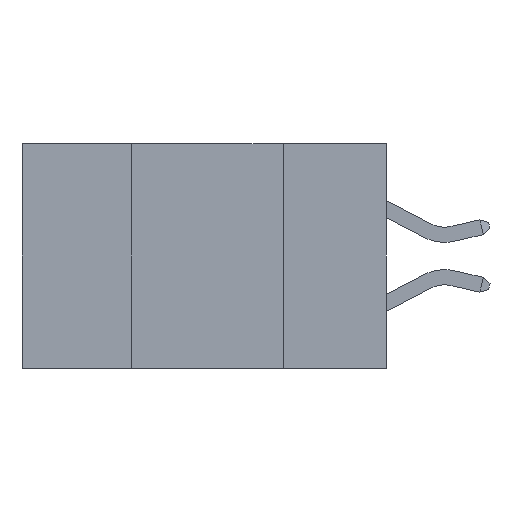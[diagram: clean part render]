
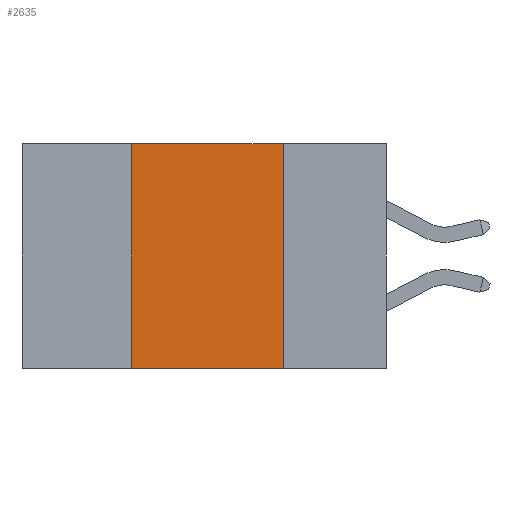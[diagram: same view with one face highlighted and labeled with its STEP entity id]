
A CAD part, left-side view. The second image highlights one B-rep face of the part: STEP entity #2635.
In plain terms, the highlighted planar face has unit normal (-1, 0, 0).
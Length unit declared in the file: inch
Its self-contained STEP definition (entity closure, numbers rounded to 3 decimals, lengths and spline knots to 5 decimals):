
#463 = EDGE_CURVE ( 'NONE', #7855, #1455, #8124, .T. ) ;
#603 = EDGE_CURVE ( 'NONE', #8532, #7855, #4372, .T. ) ;
#658 = EDGE_CURVE ( 'NONE', #8321, #8532, #3802, .T. ) ;
#676 = EDGE_CURVE ( 'NONE', #8321, #1455, #4835, .T. ) ;
#708 = ORIENTED_EDGE ( 'NONE', *, *, #603, .F. ) ;
#980 = VECTOR ( 'NONE', #6757, 39.37008 ) ;
#1153 = DIRECTION ( 'NONE',  ( 0., 0., -1. ) ) ;
#1199 = DIRECTION ( 'NONE',  ( 1., 0., 0. ) ) ;
#1331 = CARTESIAN_POINT ( 'NONE',  ( 0., 0.6, 0. ) ) ;
#1409 = PLANE ( 'NONE',  #3883 ) ;
#1455 = VERTEX_POINT ( 'NONE', #5468 ) ;
#2279 = DIRECTION ( 'NONE',  ( 0., -1., 0. ) ) ;
#2634 = VECTOR ( 'NONE', #2279, 39.37008 ) ;
#2635 = ADVANCED_FACE ( 'NONE', ( #7624 ), #1409, .F. ) ;
#2991 = CARTESIAN_POINT ( 'NONE',  ( 0., 0.42, -0.37 ) ) ;
#3249 = EDGE_LOOP ( 'NONE', ( #7687, #708, #6214, #7905 ) ) ;
#3391 = DIRECTION ( 'NONE',  ( 0., 0., 1. ) ) ;
#3802 = LINE ( 'NONE', #2991, #8303 ) ;
#3873 = CARTESIAN_POINT ( 'NONE',  ( 0., 0.17, -0.37 ) ) ;
#3883 = AXIS2_PLACEMENT_3D ( 'NONE', #1331, #1199, #1153 ) ;
#4226 = CARTESIAN_POINT ( 'NONE',  ( 0., 0.6, 0. ) ) ;
#4372 = LINE ( 'NONE', #4226, #2634 ) ;
#4380 = CARTESIAN_POINT ( 'NONE',  ( 0., 0.6, -0.37 ) ) ;
#4633 = VECTOR ( 'NONE', #7746, 39.37008 ) ;
#4835 = LINE ( 'NONE', #4380, #4633 ) ;
#5468 = CARTESIAN_POINT ( 'NONE',  ( 0., 0.17, -0.37 ) ) ;
#5821 = CARTESIAN_POINT ( 'NONE',  ( 0., 0.42, 0. ) ) ;
#6214 = ORIENTED_EDGE ( 'NONE', *, *, #658, .F. ) ;
#6749 = CARTESIAN_POINT ( 'NONE',  ( 0., 0.17, 0. ) ) ;
#6757 = DIRECTION ( 'NONE',  ( 0., 0., -1. ) ) ;
#7624 = FACE_OUTER_BOUND ( 'NONE', #3249, .T. ) ;
#7687 = ORIENTED_EDGE ( 'NONE', *, *, #463, .F. ) ;
#7746 = DIRECTION ( 'NONE',  ( 0., -1., 0. ) ) ;
#7855 = VERTEX_POINT ( 'NONE', #6749 ) ;
#7905 = ORIENTED_EDGE ( 'NONE', *, *, #676, .T. ) ;
#8124 = LINE ( 'NONE', #3873, #980 ) ;
#8241 = CARTESIAN_POINT ( 'NONE',  ( 0., 0.42, -0.37 ) ) ;
#8303 = VECTOR ( 'NONE', #3391, 39.37008 ) ;
#8321 = VERTEX_POINT ( 'NONE', #8241 ) ;
#8532 = VERTEX_POINT ( 'NONE', #5821 ) ;
